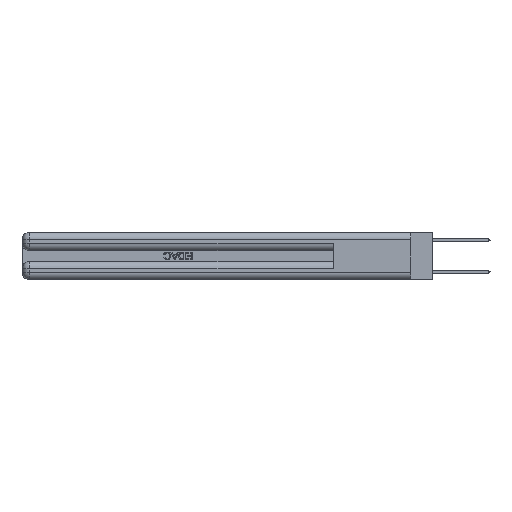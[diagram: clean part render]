
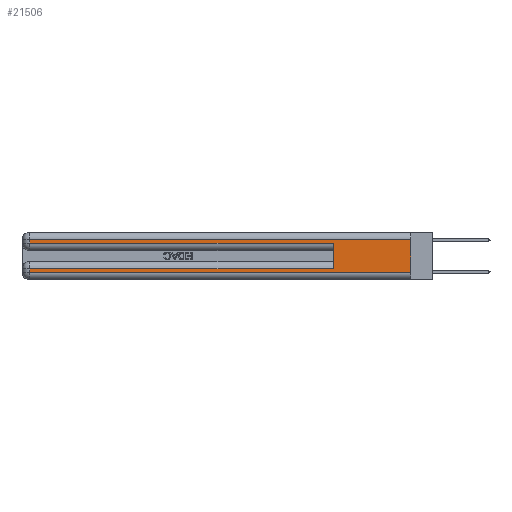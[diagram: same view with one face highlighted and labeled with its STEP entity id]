
A CAD part, left-side view. The second image highlights one B-rep face of the part: STEP entity #21506.
In plain terms, the highlighted planar face has unit normal (-1, 0, 0).
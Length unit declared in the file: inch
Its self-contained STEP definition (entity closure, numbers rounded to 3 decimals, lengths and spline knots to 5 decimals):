
#245 = VECTOR ( 'NONE', #25738, 39.37008 ) ;
#276 = DIRECTION ( 'NONE',  ( 1., 0., 0. ) ) ;
#475 = DIRECTION ( 'NONE',  ( 0., 0., -1. ) ) ;
#956 = VECTOR ( 'NONE', #15102, 39.37008 ) ;
#1958 = CARTESIAN_POINT ( 'NONE',  ( 0., 0., 0.285 ) ) ;
#2357 = CARTESIAN_POINT ( 'NONE',  ( 0., 0., 0.31 ) ) ;
#2507 = CARTESIAN_POINT ( 'NONE',  ( 0., 0., 0.31 ) ) ;
#2653 = EDGE_CURVE ( 'NONE', #31280, #27490, #16117, .T. ) ;
#2823 = EDGE_LOOP ( 'NONE', ( #29372, #11077, #18637, #13047, #17015, #16060, #20271, #25645 ) ) ;
#4229 = CARTESIAN_POINT ( 'NONE',  ( 0., 2.94, 0.37 ) ) ;
#6519 = DIRECTION ( 'NONE',  ( 0., -1., 0. ) ) ;
#6938 = EDGE_CURVE ( 'NONE', #27783, #31280, #30614, .T. ) ;
#7560 = VECTOR ( 'NONE', #26609, 39.37008 ) ;
#7627 = CARTESIAN_POINT ( 'NONE',  ( 0., 2.94, 0.37 ) ) ;
#8164 = CARTESIAN_POINT ( 'NONE',  ( 0., 0.6, 0.145 ) ) ;
#8749 = CARTESIAN_POINT ( 'NONE',  ( 0., 0.6, 0.285 ) ) ;
#8855 = VERTEX_POINT ( 'NONE', #8749 ) ;
#9484 = VERTEX_POINT ( 'NONE', #28953 ) ;
#9718 = VERTEX_POINT ( 'NONE', #32489 ) ;
#9832 = DIRECTION ( 'NONE',  ( 0., 1., 0. ) ) ;
#10522 = CARTESIAN_POINT ( 'NONE',  ( 0., 0., 0.37 ) ) ;
#10683 = LINE ( 'NONE', #20897, #15151 ) ;
#11077 = ORIENTED_EDGE ( 'NONE', *, *, #24500, .T. ) ;
#12181 = LINE ( 'NONE', #2357, #30184 ) ;
#12471 = VECTOR ( 'NONE', #6519, 39.37008 ) ;
#12829 = EDGE_CURVE ( 'NONE', #24699, #27490, #13044, .T. ) ;
#12841 = CARTESIAN_POINT ( 'NONE',  ( 0., 2.94, 0.31 ) ) ;
#13044 = LINE ( 'NONE', #10522, #245 ) ;
#13047 = ORIENTED_EDGE ( 'NONE', *, *, #30404, .T. ) ;
#13140 = DIRECTION ( 'NONE',  ( 0., 0., -1. ) ) ;
#14884 = EDGE_CURVE ( 'NONE', #9484, #27783, #10683, .T. ) ;
#15102 = DIRECTION ( 'NONE',  ( 0., -1., 0. ) ) ;
#15151 = VECTOR ( 'NONE', #18052, 39.37008 ) ;
#16060 = ORIENTED_EDGE ( 'NONE', *, *, #14884, .T. ) ;
#16117 = LINE ( 'NONE', #29517, #12471 ) ;
#16461 = AXIS2_PLACEMENT_3D ( 'NONE', #23662, #276, #13140 ) ;
#17015 = ORIENTED_EDGE ( 'NONE', *, *, #19827, .F. ) ;
#17494 = EDGE_CURVE ( 'NONE', #31515, #9718, #29631, .T. ) ;
#17786 = CARTESIAN_POINT ( 'NONE',  ( 0., 0., 0.06 ) ) ;
#18052 = DIRECTION ( 'NONE',  ( 0., 1., 0. ) ) ;
#18637 = ORIENTED_EDGE ( 'NONE', *, *, #17494, .T. ) ;
#19827 = EDGE_CURVE ( 'NONE', #9484, #8855, #29153, .T. ) ;
#20271 = ORIENTED_EDGE ( 'NONE', *, *, #6938, .T. ) ;
#20897 = CARTESIAN_POINT ( 'NONE',  ( 0., 0., 0.085 ) ) ;
#21003 = FACE_OUTER_BOUND ( 'NONE', #2823, .T. ) ;
#21091 = CARTESIAN_POINT ( 'NONE',  ( 0., 2.94, 0.06 ) ) ;
#21506 = ADVANCED_FACE ( 'NONE', ( #21003 ), #26169, .F. ) ;
#21759 = DIRECTION ( 'NONE',  ( 0., 0., -1. ) ) ;
#22773 = VECTOR ( 'NONE', #475, 39.37008 ) ;
#23662 = CARTESIAN_POINT ( 'NONE',  ( 0., 0., 0.37 ) ) ;
#24500 = EDGE_CURVE ( 'NONE', #24699, #31515, #12181, .T. ) ;
#24699 = VERTEX_POINT ( 'NONE', #2507 ) ;
#25645 = ORIENTED_EDGE ( 'NONE', *, *, #2653, .T. ) ;
#25738 = DIRECTION ( 'NONE',  ( 0., 0., -1. ) ) ;
#26169 = PLANE ( 'NONE',  #16461 ) ;
#26609 = DIRECTION ( 'NONE',  ( 0., 0., 1. ) ) ;
#27490 = VERTEX_POINT ( 'NONE', #17786 ) ;
#27783 = VERTEX_POINT ( 'NONE', #29847 ) ;
#27987 = VECTOR ( 'NONE', #21759, 39.37008 ) ;
#28953 = CARTESIAN_POINT ( 'NONE',  ( 0., 0.6, 0.085 ) ) ;
#29153 = LINE ( 'NONE', #8164, #7560 ) ;
#29372 = ORIENTED_EDGE ( 'NONE', *, *, #12829, .F. ) ;
#29517 = CARTESIAN_POINT ( 'NONE',  ( 0., 0., 0.06 ) ) ;
#29631 = LINE ( 'NONE', #4229, #27987 ) ;
#29847 = CARTESIAN_POINT ( 'NONE',  ( 0., 2.94, 0.085 ) ) ;
#30184 = VECTOR ( 'NONE', #9832, 39.37008 ) ;
#30404 = EDGE_CURVE ( 'NONE', #9718, #8855, #32879, .T. ) ;
#30614 = LINE ( 'NONE', #7627, #22773 ) ;
#31280 = VERTEX_POINT ( 'NONE', #21091 ) ;
#31515 = VERTEX_POINT ( 'NONE', #12841 ) ;
#32489 = CARTESIAN_POINT ( 'NONE',  ( 0., 2.94, 0.285 ) ) ;
#32879 = LINE ( 'NONE', #1958, #956 ) ;
